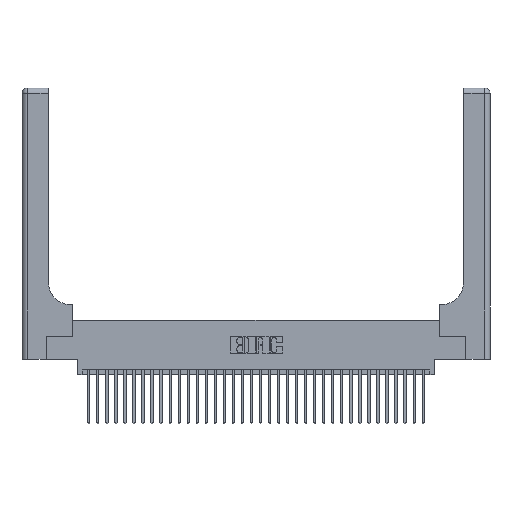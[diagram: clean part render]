
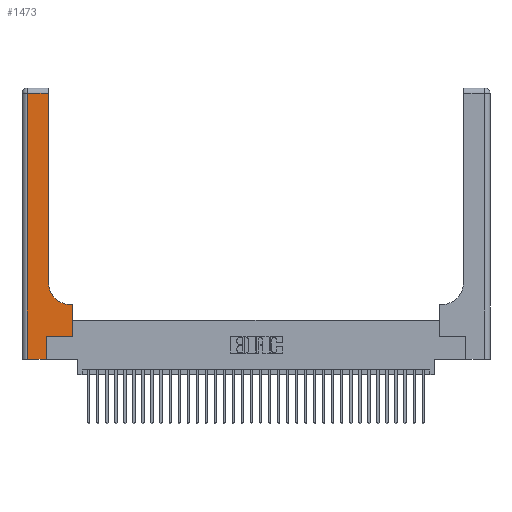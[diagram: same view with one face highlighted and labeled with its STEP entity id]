
A CAD part, top view. The second image highlights one B-rep face of the part: STEP entity #1473.
In plain terms, the highlighted planar face has unit normal (0, 0, 1).
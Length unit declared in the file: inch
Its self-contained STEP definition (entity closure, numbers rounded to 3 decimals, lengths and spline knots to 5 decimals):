
#293 = DIRECTION ( 'NONE',  ( 1., 0., 0. ) ) ;
#398 = ORIENTED_EDGE ( 'NONE', *, *, #5455, .T. ) ;
#897 = VECTOR ( 'NONE', #28371, 39.37008 ) ;
#1072 = CARTESIAN_POINT ( 'NONE',  ( 0.269, 0.25, 0.37 ) ) ;
#1334 = DIRECTION ( 'NONE',  ( -1., 0., 0. ) ) ;
#1473 = ADVANCED_FACE ( 'NONE', ( #8178 ), #7342, .F. ) ;
#1736 = LINE ( 'NONE', #10073, #2622 ) ;
#2622 = VECTOR ( 'NONE', #20858, 39.37008 ) ;
#4082 = ORIENTED_EDGE ( 'NONE', *, *, #12928, .T. ) ;
#4139 = EDGE_CURVE ( 'NONE', #19256, #6252, #10113, .T. ) ;
#4294 = LINE ( 'NONE', #11426, #21525 ) ;
#4670 = VECTOR ( 'NONE', #15185, 39.37008 ) ;
#5096 = CARTESIAN_POINT ( 'NONE',  ( 0.2915, 2.94, 0.37 ) ) ;
#5120 = LINE ( 'NONE', #15099, #11606 ) ;
#5455 = EDGE_CURVE ( 'NONE', #19488, #27927, #22854, .T. ) ;
#6252 = VERTEX_POINT ( 'NONE', #26889 ) ;
#6394 = CARTESIAN_POINT ( 'NONE',  ( 0.269, 0., 0.37 ) ) ;
#6481 = CARTESIAN_POINT ( 'NONE',  ( 0.5415, 0.85, 0.37 ) ) ;
#6841 = VECTOR ( 'NONE', #11052, 39.37008 ) ;
#7069 = EDGE_LOOP ( 'NONE', ( #30569, #21764, #398, #17254, #26777, #4082, #31837, #22597, #22903 ) ) ;
#7342 = PLANE ( 'NONE',  #26323 ) ;
#8127 = LINE ( 'NONE', #21591, #6841 ) ;
#8178 = FACE_OUTER_BOUND ( 'NONE', #7069, .T. ) ;
#8623 = EDGE_CURVE ( 'NONE', #26699, #35710, #8127, .T. ) ;
#8975 = EDGE_CURVE ( 'NONE', #6252, #19855, #21885, .T. ) ;
#9436 = CARTESIAN_POINT ( 'NONE',  ( 0.2915, 3., 0.37 ) ) ;
#10073 = CARTESIAN_POINT ( 'NONE',  ( 0.269, 0.25, 0.37 ) ) ;
#10113 = CIRCLE ( 'NONE', #28886, 0.25 ) ;
#10244 = DIRECTION ( 'NONE',  ( 0., 0., -1. ) ) ;
#10252 = CARTESIAN_POINT ( 'NONE',  ( 0.5585, 0.6, 0.37 ) ) ;
#11052 = DIRECTION ( 'NONE',  ( 0., 1., 0. ) ) ;
#11426 = CARTESIAN_POINT ( 'NONE',  ( 0., 0., 0.37 ) ) ;
#11606 = VECTOR ( 'NONE', #1334, 39.37008 ) ;
#12134 = DIRECTION ( 'NONE',  ( 0., 0., -1. ) ) ;
#12210 = DIRECTION ( 'NONE',  ( 0., 1., 0. ) ) ;
#12928 = EDGE_CURVE ( 'NONE', #26529, #26699, #1736, .T. ) ;
#13198 = VECTOR ( 'NONE', #35037, 39.37008 ) ;
#15099 = CARTESIAN_POINT ( 'NONE',  ( 0.2915, 0.6, 0.37 ) ) ;
#15185 = DIRECTION ( 'NONE',  ( -1., 0., 0. ) ) ;
#15500 = DIRECTION ( 'NONE',  ( 1., 0., 0. ) ) ;
#15649 = DIRECTION ( 'NONE',  ( -1., 0., 0. ) ) ;
#17254 = ORIENTED_EDGE ( 'NONE', *, *, #20803, .T. ) ;
#17375 = EDGE_CURVE ( 'NONE', #19855, #19488, #28756, .T. ) ;
#18426 = VECTOR ( 'NONE', #12210, 39.37008 ) ;
#19256 = VERTEX_POINT ( 'NONE', #26132 ) ;
#19488 = VERTEX_POINT ( 'NONE', #27068 ) ;
#19631 = LINE ( 'NONE', #29078, #13198 ) ;
#19665 = VERTEX_POINT ( 'NONE', #6394 ) ;
#19855 = VERTEX_POINT ( 'NONE', #5096 ) ;
#20803 = EDGE_CURVE ( 'NONE', #27927, #19665, #4294, .T. ) ;
#20858 = DIRECTION ( 'NONE',  ( 1., 0., 0. ) ) ;
#20874 = CARTESIAN_POINT ( 'NONE',  ( 0., 2.94, 0.37 ) ) ;
#21151 = CARTESIAN_POINT ( 'NONE',  ( 0., 3., 0.37 ) ) ;
#21525 = VECTOR ( 'NONE', #293, 39.37008 ) ;
#21543 = CARTESIAN_POINT ( 'NONE',  ( 0.5585, 0.25, 0.37 ) ) ;
#21591 = CARTESIAN_POINT ( 'NONE',  ( 0.5585, 0.25, 0.37 ) ) ;
#21764 = ORIENTED_EDGE ( 'NONE', *, *, #17375, .T. ) ;
#21885 = LINE ( 'NONE', #9436, #18426 ) ;
#22597 = ORIENTED_EDGE ( 'NONE', *, *, #33322, .T. ) ;
#22854 = LINE ( 'NONE', #31047, #897 ) ;
#22903 = ORIENTED_EDGE ( 'NONE', *, *, #4139, .T. ) ;
#23526 = EDGE_CURVE ( 'NONE', #19665, #26529, #19631, .T. ) ;
#26132 = CARTESIAN_POINT ( 'NONE',  ( 0.5415, 0.6, 0.37 ) ) ;
#26323 = AXIS2_PLACEMENT_3D ( 'NONE', #21151, #10244, #15649 ) ;
#26529 = VERTEX_POINT ( 'NONE', #1072 ) ;
#26531 = CARTESIAN_POINT ( 'NONE',  ( 0.06, 0., 0.37 ) ) ;
#26699 = VERTEX_POINT ( 'NONE', #21543 ) ;
#26777 = ORIENTED_EDGE ( 'NONE', *, *, #23526, .T. ) ;
#26889 = CARTESIAN_POINT ( 'NONE',  ( 0.2915, 0.85, 0.37 ) ) ;
#27068 = CARTESIAN_POINT ( 'NONE',  ( 0.06, 2.94, 0.37 ) ) ;
#27927 = VERTEX_POINT ( 'NONE', #26531 ) ;
#28371 = DIRECTION ( 'NONE',  ( 0., -1., 0. ) ) ;
#28756 = LINE ( 'NONE', #20874, #4670 ) ;
#28886 = AXIS2_PLACEMENT_3D ( 'NONE', #6481, #12134, #15500 ) ;
#29078 = CARTESIAN_POINT ( 'NONE',  ( 0.269, 0., 0.37 ) ) ;
#30569 = ORIENTED_EDGE ( 'NONE', *, *, #8975, .T. ) ;
#31047 = CARTESIAN_POINT ( 'NONE',  ( 0.06, 3., 0.37 ) ) ;
#31837 = ORIENTED_EDGE ( 'NONE', *, *, #8623, .T. ) ;
#33322 = EDGE_CURVE ( 'NONE', #35710, #19256, #5120, .T. ) ;
#35037 = DIRECTION ( 'NONE',  ( 0., 1., 0. ) ) ;
#35710 = VERTEX_POINT ( 'NONE', #10252 ) ;
